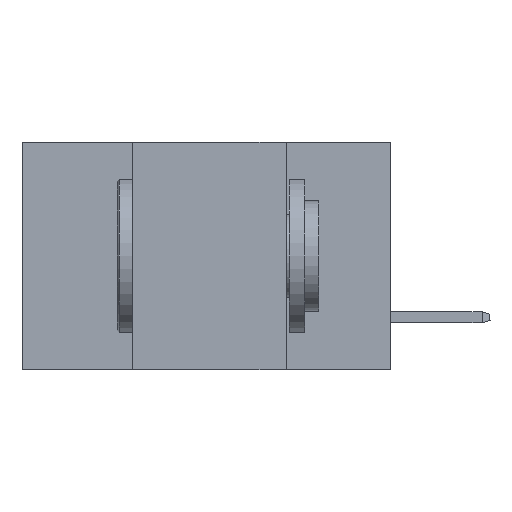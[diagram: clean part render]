
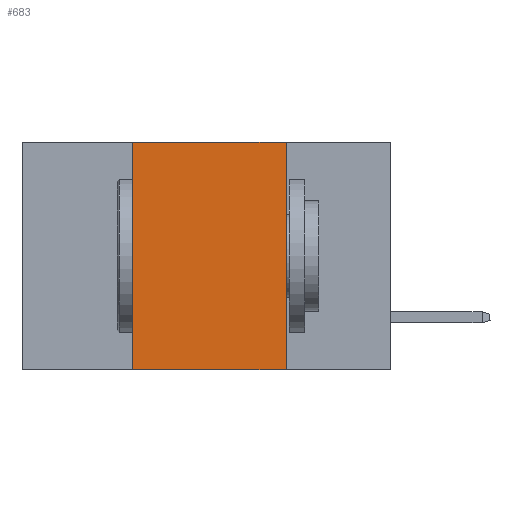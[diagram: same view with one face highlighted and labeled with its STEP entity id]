
A CAD part, left-side view. The second image highlights one B-rep face of the part: STEP entity #683.
In plain terms, the highlighted planar face has unit normal (-1, 0, 0).
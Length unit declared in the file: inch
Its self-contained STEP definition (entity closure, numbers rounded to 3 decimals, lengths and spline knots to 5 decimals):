
#35 = LINE ( 'NONE', #7058, #9853 ) ;
#179 = DIRECTION ( 'NONE',  ( 0., 0., -1. ) ) ;
#653 = LINE ( 'NONE', #10201, #3590 ) ;
#683 = ADVANCED_FACE ( 'NONE', ( #10650 ), #14271, .F. ) ;
#963 = CARTESIAN_POINT ( 'NONE',  ( 0., 0.6, 0. ) ) ;
#3590 = VECTOR ( 'NONE', #4820, 39.37008 ) ;
#3832 = EDGE_CURVE ( 'NONE', #11536, #21777, #653, .T. ) ;
#4820 = DIRECTION ( 'NONE',  ( 0., 0., 1. ) ) ;
#4955 = EDGE_LOOP ( 'NONE', ( #6009, #20414, #13397, #5398 ) ) ;
#5398 = ORIENTED_EDGE ( 'NONE', *, *, #7317, .T. ) ;
#6009 = ORIENTED_EDGE ( 'NONE', *, *, #18630, .F. ) ;
#6086 = DIRECTION ( 'NONE',  ( 1., 0., 0. ) ) ;
#6203 = CARTESIAN_POINT ( 'NONE',  ( 0., 0.17, 0. ) ) ;
#6459 = VERTEX_POINT ( 'NONE', #14342 ) ;
#7023 = VERTEX_POINT ( 'NONE', #6203 ) ;
#7058 = CARTESIAN_POINT ( 'NONE',  ( 0., 0.17, 0. ) ) ;
#7317 = EDGE_CURVE ( 'NONE', #11536, #6459, #19448, .T. ) ;
#7642 = DIRECTION ( 'NONE',  ( 0., 0., -1. ) ) ;
#9848 = VECTOR ( 'NONE', #11513, 39.37008 ) ;
#9853 = VECTOR ( 'NONE', #179, 39.37008 ) ;
#9898 = VECTOR ( 'NONE', #19624, 39.37008 ) ;
#10201 = CARTESIAN_POINT ( 'NONE',  ( 0., 0.42, 0. ) ) ;
#10650 = FACE_OUTER_BOUND ( 'NONE', #4955, .T. ) ;
#11513 = DIRECTION ( 'NONE',  ( 0., -1., 0. ) ) ;
#11536 = VERTEX_POINT ( 'NONE', #19387 ) ;
#13106 = CARTESIAN_POINT ( 'NONE',  ( 0., 0.42, 0. ) ) ;
#13397 = ORIENTED_EDGE ( 'NONE', *, *, #3832, .F. ) ;
#14271 = PLANE ( 'NONE',  #19192 ) ;
#14342 = CARTESIAN_POINT ( 'NONE',  ( 0., 0.17, -0.37 ) ) ;
#14972 = EDGE_CURVE ( 'NONE', #21777, #7023, #16998, .T. ) ;
#16998 = LINE ( 'NONE', #963, #9848 ) ;
#17772 = CARTESIAN_POINT ( 'NONE',  ( 0., 0.6, 0. ) ) ;
#18630 = EDGE_CURVE ( 'NONE', #7023, #6459, #35, .T. ) ;
#19192 = AXIS2_PLACEMENT_3D ( 'NONE', #17772, #6086, #7642 ) ;
#19387 = CARTESIAN_POINT ( 'NONE',  ( 0., 0.42, -0.37 ) ) ;
#19448 = LINE ( 'NONE', #21008, #9898 ) ;
#19624 = DIRECTION ( 'NONE',  ( 0., -1., 0. ) ) ;
#20414 = ORIENTED_EDGE ( 'NONE', *, *, #14972, .F. ) ;
#21008 = CARTESIAN_POINT ( 'NONE',  ( 0., 0.6, -0.37 ) ) ;
#21777 = VERTEX_POINT ( 'NONE', #13106 ) ;
